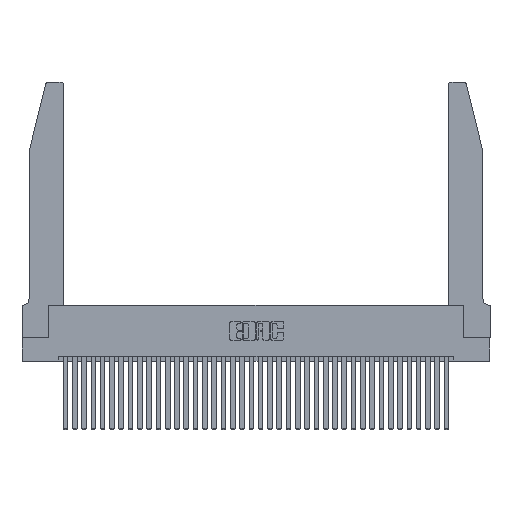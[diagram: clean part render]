
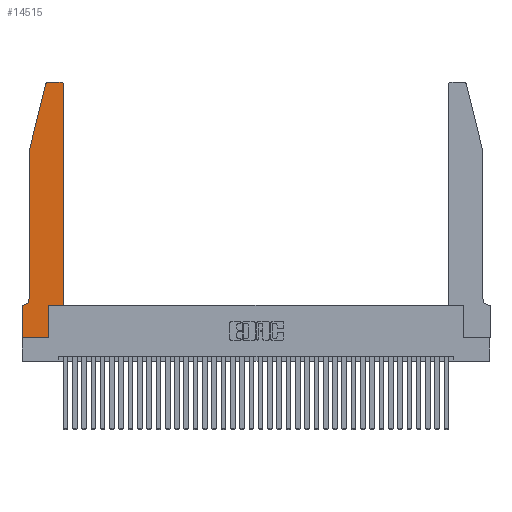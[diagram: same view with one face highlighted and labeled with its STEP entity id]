
A CAD part, top view. The second image highlights one B-rep face of the part: STEP entity #14515.
In plain terms, the highlighted planar face has unit normal (0, 0, 1).
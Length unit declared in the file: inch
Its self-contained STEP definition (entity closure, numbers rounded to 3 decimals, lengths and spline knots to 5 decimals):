
#44 = CARTESIAN_POINT ( 'NONE',  ( 0.0755, 2., 0.37 ) ) ;
#453 = LINE ( 'NONE', #31660, #31718 ) ;
#1157 = EDGE_CURVE ( 'NONE', #20911, #4991, #35828, .T. ) ;
#1188 = AXIS2_PLACEMENT_3D ( 'NONE', #27036, #29935, #15338 ) ;
#1302 = VERTEX_POINT ( 'NONE', #22760 ) ;
#2076 = DIRECTION ( 'NONE',  ( 1., 0., 0. ) ) ;
#2132 = PLANE ( 'NONE',  #35012 ) ;
#2170 = DIRECTION ( 'NONE',  ( 0., 0., -1. ) ) ;
#2734 = DIRECTION ( 'NONE',  ( 0., -1., 0. ) ) ;
#2879 = VECTOR ( 'NONE', #2734, 39.37008 ) ;
#2915 = EDGE_CURVE ( 'NONE', #1302, #4233, #14209, .T. ) ;
#2969 = VERTEX_POINT ( 'NONE', #34917 ) ;
#3408 = VERTEX_POINT ( 'NONE', #30295 ) ;
#3819 = EDGE_CURVE ( 'NONE', #3408, #29358, #7793, .T. ) ;
#3857 = VECTOR ( 'NONE', #36396, 39.37008 ) ;
#3892 = EDGE_CURVE ( 'NONE', #7866, #4893, #29488, .T. ) ;
#4233 = VERTEX_POINT ( 'NONE', #11530 ) ;
#4351 = ORIENTED_EDGE ( 'NONE', *, *, #33696, .T. ) ;
#4893 = VERTEX_POINT ( 'NONE', #13978 ) ;
#4991 = VERTEX_POINT ( 'NONE', #6278 ) ;
#5869 = CARTESIAN_POINT ( 'NONE',  ( 0.4505, 0.35, 0.37 ) ) ;
#6103 = CARTESIAN_POINT ( 'NONE',  ( 0.4505, 2.72, 0.37 ) ) ;
#6190 = EDGE_CURVE ( 'NONE', #2969, #33632, #26608, .T. ) ;
#6278 = CARTESIAN_POINT ( 'NONE',  ( 0.4205, 2.75, 0.37 ) ) ;
#6386 = EDGE_LOOP ( 'NONE', ( #4351, #14735, #33954, #21595, #16001, #6816, #20559, #35646, #15749, #22151, #16670, #13132 ) ) ;
#6816 = ORIENTED_EDGE ( 'NONE', *, *, #3819, .T. ) ;
#7793 = LINE ( 'NONE', #28591, #8230 ) ;
#7866 = VERTEX_POINT ( 'NONE', #10483 ) ;
#8230 = VECTOR ( 'NONE', #20135, 39.37008 ) ;
#8486 = VERTEX_POINT ( 'NONE', #32062 ) ;
#9104 = LINE ( 'NONE', #18263, #12709 ) ;
#10483 = CARTESIAN_POINT ( 'NONE',  ( 0.25487, 2.72718, 0.37 ) ) ;
#10904 = EDGE_CURVE ( 'NONE', #29358, #2969, #36559, .T. ) ;
#11479 = VECTOR ( 'NONE', #12911, 39.37008 ) ;
#11530 = CARTESIAN_POINT ( 'NONE',  ( 0.4505, 0.35, 0.37 ) ) ;
#12709 = VECTOR ( 'NONE', #13198, 39.37008 ) ;
#12911 = DIRECTION ( 'NONE',  ( -1., 0., 0. ) ) ;
#12971 = EDGE_CURVE ( 'NONE', #4233, #20911, #9104, .T. ) ;
#13132 = ORIENTED_EDGE ( 'NONE', *, *, #1157, .T. ) ;
#13198 = DIRECTION ( 'NONE',  ( 0., 1., 0. ) ) ;
#13327 = VERTEX_POINT ( 'NONE', #23730 ) ;
#13978 = CARTESIAN_POINT ( 'NONE',  ( 0.0755, 2., 0.37 ) ) ;
#14099 = VECTOR ( 'NONE', #28885, 39.37008 ) ;
#14209 = LINE ( 'NONE', #5869, #19646 ) ;
#14515 = ADVANCED_FACE ( 'NONE', ( #31277 ), #2132, .T. ) ;
#14735 = ORIENTED_EDGE ( 'NONE', *, *, #16477, .T. ) ;
#15208 = CARTESIAN_POINT ( 'NONE',  ( 0., 0., 0.37 ) ) ;
#15338 = DIRECTION ( 'NONE',  ( 1., 0., 0. ) ) ;
#15749 = ORIENTED_EDGE ( 'NONE', *, *, #24854, .T. ) ;
#15783 = CARTESIAN_POINT ( 'NONE',  ( 0., 0., 0.37 ) ) ;
#16001 = ORIENTED_EDGE ( 'NONE', *, *, #29813, .T. ) ;
#16205 = DIRECTION ( 'NONE',  ( 1., 0., 0. ) ) ;
#16250 = AXIS2_PLACEMENT_3D ( 'NONE', #33226, #21578, #16205 ) ;
#16399 = DIRECTION ( 'NONE',  ( 0., 0., 1. ) ) ;
#16477 = EDGE_CURVE ( 'NONE', #8486, #7866, #27694, .T. ) ;
#16670 = ORIENTED_EDGE ( 'NONE', *, *, #12971, .T. ) ;
#17629 = CARTESIAN_POINT ( 'NONE',  ( 0.0755, 2., 0.37 ) ) ;
#18263 = CARTESIAN_POINT ( 'NONE',  ( 0.4505, 0.35, 0.37 ) ) ;
#19646 = VECTOR ( 'NONE', #26164, 39.37008 ) ;
#20135 = DIRECTION ( 'NONE',  ( -1., 0., 0. ) ) ;
#20537 = LINE ( 'NONE', #24744, #11479 ) ;
#20559 = ORIENTED_EDGE ( 'NONE', *, *, #10904, .T. ) ;
#20911 = VERTEX_POINT ( 'NONE', #6103 ) ;
#21279 = EDGE_CURVE ( 'NONE', #4893, #13327, #37365, .T. ) ;
#21382 = CARTESIAN_POINT ( 'NONE',  ( 0., 0.35, 0.37 ) ) ;
#21578 = DIRECTION ( 'NONE',  ( 0., 0., 1. ) ) ;
#21595 = ORIENTED_EDGE ( 'NONE', *, *, #21279, .T. ) ;
#22151 = ORIENTED_EDGE ( 'NONE', *, *, #2915, .T. ) ;
#22579 = DIRECTION ( 'NONE',  ( 0., 1., 0. ) ) ;
#22760 = CARTESIAN_POINT ( 'NONE',  ( 0.2865, 0.35, 0.37 ) ) ;
#22908 = CARTESIAN_POINT ( 'NONE',  ( 0., 0.35, 0.37 ) ) ;
#23730 = CARTESIAN_POINT ( 'NONE',  ( 0.0755, 0.42, 0.37 ) ) ;
#24744 = CARTESIAN_POINT ( 'NONE',  ( 0.2605, 2.75, 0.37 ) ) ;
#24854 = EDGE_CURVE ( 'NONE', #33632, #1302, #453, .T. ) ;
#26164 = DIRECTION ( 'NONE',  ( 1., 0., 0. ) ) ;
#26608 = LINE ( 'NONE', #15208, #36161 ) ;
#27036 = CARTESIAN_POINT ( 'NONE',  ( 0.4205, 2.72, 0.37 ) ) ;
#27694 = CIRCLE ( 'NONE', #16250, 0.03 ) ;
#27744 = CARTESIAN_POINT ( 'NONE',  ( 0.0055, 0.42, 0.37 ) ) ;
#28591 = CARTESIAN_POINT ( 'NONE',  ( 0.0755, 0.35, 0.37 ) ) ;
#28885 = DIRECTION ( 'NONE',  ( -0.239, -0.971, 0. ) ) ;
#29358 = VERTEX_POINT ( 'NONE', #22908 ) ;
#29488 = LINE ( 'NONE', #44, #14099 ) ;
#29813 = EDGE_CURVE ( 'NONE', #13327, #3408, #34436, .T. ) ;
#29935 = DIRECTION ( 'NONE',  ( 0., 0., 1. ) ) ;
#30295 = CARTESIAN_POINT ( 'NONE',  ( 0.0055, 0.35, 0.37 ) ) ;
#31277 = FACE_OUTER_BOUND ( 'NONE', #6386, .T. ) ;
#31660 = CARTESIAN_POINT ( 'NONE',  ( 0.2865, 0.35, 0.37 ) ) ;
#31718 = VECTOR ( 'NONE', #22579, 39.37008 ) ;
#32062 = CARTESIAN_POINT ( 'NONE',  ( 0.284, 2.75, 0.37 ) ) ;
#32082 = CARTESIAN_POINT ( 'NONE',  ( 0.2865, 0., 0.37 ) ) ;
#33226 = CARTESIAN_POINT ( 'NONE',  ( 0.284, 2.72, 0.37 ) ) ;
#33521 = DIRECTION ( 'NONE',  ( 1., 0., 0. ) ) ;
#33632 = VERTEX_POINT ( 'NONE', #32082 ) ;
#33696 = EDGE_CURVE ( 'NONE', #4991, #8486, #20537, .T. ) ;
#33865 = DIRECTION ( 'NONE',  ( -1., 0., 0. ) ) ;
#33954 = ORIENTED_EDGE ( 'NONE', *, *, #3892, .T. ) ;
#34436 = CIRCLE ( 'NONE', #36903, 0.07 ) ;
#34917 = CARTESIAN_POINT ( 'NONE',  ( 0., 0., 0.37 ) ) ;
#35012 = AXIS2_PLACEMENT_3D ( 'NONE', #21382, #16399, #33521 ) ;
#35646 = ORIENTED_EDGE ( 'NONE', *, *, #6190, .T. ) ;
#35828 = CIRCLE ( 'NONE', #1188, 0.03 ) ;
#36161 = VECTOR ( 'NONE', #2076, 39.37008 ) ;
#36396 = DIRECTION ( 'NONE',  ( 0., -1., 0. ) ) ;
#36559 = LINE ( 'NONE', #15783, #3857 ) ;
#36903 = AXIS2_PLACEMENT_3D ( 'NONE', #27744, #2170, #33865 ) ;
#37365 = LINE ( 'NONE', #17629, #2879 ) ;
